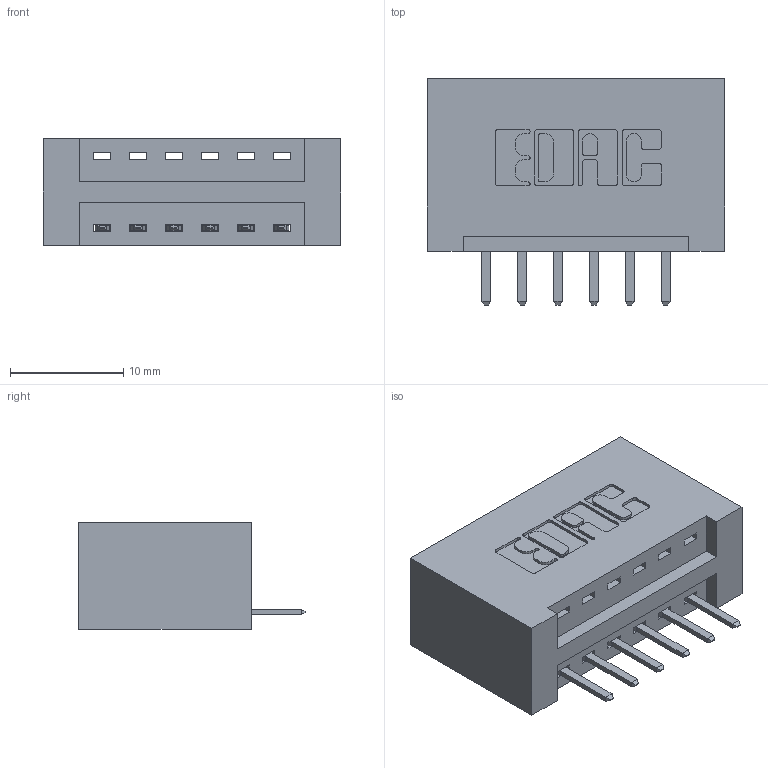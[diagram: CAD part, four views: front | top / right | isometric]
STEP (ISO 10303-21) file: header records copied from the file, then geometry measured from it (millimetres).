
FILE_DESCRIPTION (( 'STEP AP203' ), '1' );
FILE_NAME ('396-006-520-101.STEP', '2018-08-30T22:34:52', ( '' ), ( '' ), 'SwSTEP 2.0', 'SolidWorks 2016', '' );
FILE_SCHEMA (( 'CONFIG_CONTROL_DESIGN' ));
Length unit declared in the file: inch
Products named in the file (3): 346 Part_No Mounting Lugs; 345-292-001_345-293-120; 396-006-520-101
Assembly tree (7 placements, depth 2):
  396-006-520-101
    346 Part_No Mounting Lugs
    345-292-001_345-293-120  x6
Bounding box: 26.29 x 20.02 x 9.4 mm (x, y, z)
Volume: 2800.6 mm3; surface area: 3129.3 mm2
Topology: 7 solids, 7 shells, 486 faces, 1409 edges, 922 vertices
Faces by surface type: plane 324, cylinder 162
Entity records: 8407 total; most frequent: CARTESIAN_POINT 1470, ORIENTED_EDGE 1398, DIRECTION 1323, EDGE_CURVE 699, LINE 547, VECTOR 547, VERTEX_POINT 462, AXIS2_PLACEMENT_3D 388
